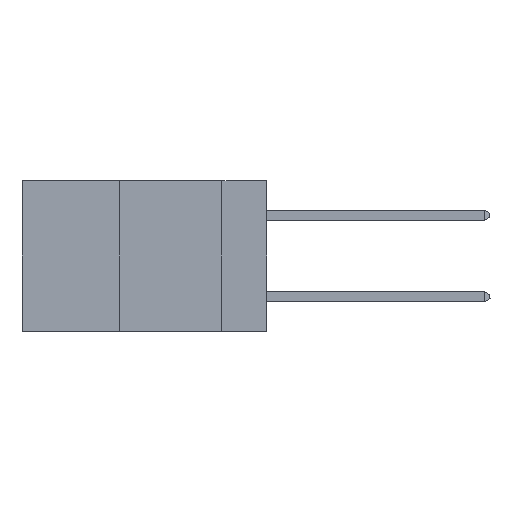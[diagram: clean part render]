
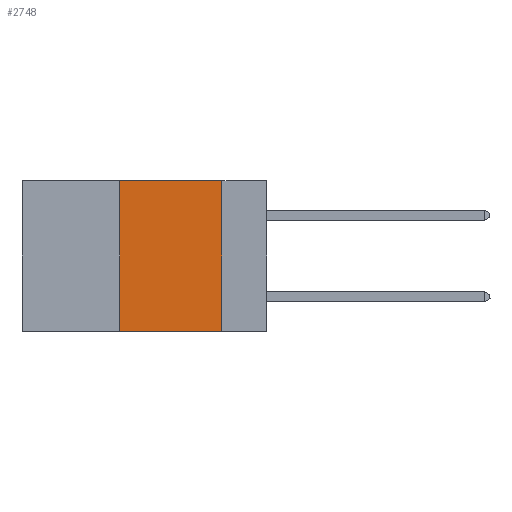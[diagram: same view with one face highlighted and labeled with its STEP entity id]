
A CAD part, left-side view. The second image highlights one B-rep face of the part: STEP entity #2748.
In plain terms, the highlighted planar face has unit normal (-1, 0, 0).
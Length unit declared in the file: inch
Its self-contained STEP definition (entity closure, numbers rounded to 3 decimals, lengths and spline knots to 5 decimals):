
#538 = CARTESIAN_POINT ( 'NONE',  ( 0., 0.36, -0.37 ) ) ;
#993 = VERTEX_POINT ( 'NONE', #15670 ) ;
#2748 = ADVANCED_FACE ( 'NONE', ( #19158 ), #6093, .F. ) ;
#3093 = CARTESIAN_POINT ( 'NONE',  ( 0., 0.11, 0. ) ) ;
#3862 = ORIENTED_EDGE ( 'NONE', *, *, #15591, .T. ) ;
#3895 = ORIENTED_EDGE ( 'NONE', *, *, #10017, .F. ) ;
#3909 = CARTESIAN_POINT ( 'NONE',  ( 0., 0.11, -0.37 ) ) ;
#4614 = DIRECTION ( 'NONE',  ( 0., 0., -1. ) ) ;
#5811 = LINE ( 'NONE', #8488, #7122 ) ;
#5860 = VERTEX_POINT ( 'NONE', #6703 ) ;
#6093 = PLANE ( 'NONE',  #8862 ) ;
#6393 = DIRECTION ( 'NONE',  ( 1., 0., 0. ) ) ;
#6674 = EDGE_CURVE ( 'NONE', #993, #21368, #13365, .T. ) ;
#6703 = CARTESIAN_POINT ( 'NONE',  ( 0., 0.36, 0. ) ) ;
#6883 = VECTOR ( 'NONE', #9717, 39.37008 ) ;
#6981 = DIRECTION ( 'NONE',  ( 0., -1., 0. ) ) ;
#7122 = VECTOR ( 'NONE', #6981, 39.37008 ) ;
#8025 = VERTEX_POINT ( 'NONE', #538 ) ;
#8488 = CARTESIAN_POINT ( 'NONE',  ( 0., 0.6, 0. ) ) ;
#8661 = DIRECTION ( 'NONE',  ( 0., 0., 1. ) ) ;
#8862 = AXIS2_PLACEMENT_3D ( 'NONE', #9558, #6393, #4614 ) ;
#9558 = CARTESIAN_POINT ( 'NONE',  ( 0., 0.6, 0. ) ) ;
#9717 = DIRECTION ( 'NONE',  ( 0., -1., 0. ) ) ;
#9890 = VECTOR ( 'NONE', #8661, 39.37008 ) ;
#10017 = EDGE_CURVE ( 'NONE', #5860, #993, #5811, .T. ) ;
#11682 = LINE ( 'NONE', #19982, #6883 ) ;
#13365 = LINE ( 'NONE', #3093, #20044 ) ;
#13930 = EDGE_CURVE ( 'NONE', #8025, #5860, #17898, .T. ) ;
#15507 = CARTESIAN_POINT ( 'NONE',  ( 0., 0.36, 0. ) ) ;
#15591 = EDGE_CURVE ( 'NONE', #8025, #21368, #11682, .T. ) ;
#15670 = CARTESIAN_POINT ( 'NONE',  ( 0., 0.11, 0. ) ) ;
#16409 = EDGE_LOOP ( 'NONE', ( #19762, #3895, #21354, #3862 ) ) ;
#16695 = DIRECTION ( 'NONE',  ( 0., 0., -1. ) ) ;
#17898 = LINE ( 'NONE', #15507, #9890 ) ;
#19158 = FACE_OUTER_BOUND ( 'NONE', #16409, .T. ) ;
#19762 = ORIENTED_EDGE ( 'NONE', *, *, #6674, .F. ) ;
#19982 = CARTESIAN_POINT ( 'NONE',  ( 0., 0.6, -0.37 ) ) ;
#20044 = VECTOR ( 'NONE', #16695, 39.37008 ) ;
#21354 = ORIENTED_EDGE ( 'NONE', *, *, #13930, .F. ) ;
#21368 = VERTEX_POINT ( 'NONE', #3909 ) ;
